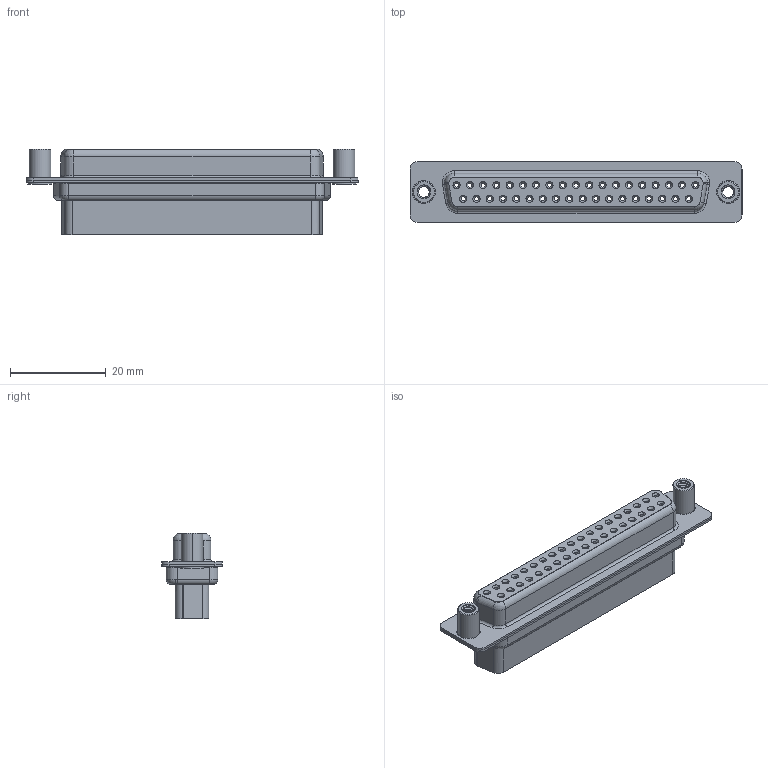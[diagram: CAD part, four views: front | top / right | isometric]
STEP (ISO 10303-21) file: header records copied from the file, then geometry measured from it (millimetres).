
FILE_DESCRIPTION (( 'STEP AP203' ), '1' );
FILE_NAME ('628-050-010-330.STEP', '2018-11-21T22:18:59', ( '' ), ( '' ), 'SwSTEP 2.0', 'SolidWorks 2016', '' );
FILE_SCHEMA (( 'CONFIG_CONTROL_DESIGN' ));
Length unit declared in the file: millimetre
Products named in the file (5): 628 Housing_37 HP; 628 Shell Front_37 Contacts; 628 Shell Rear_37 Contacts; 628 4-40 Threaded Standoff; 628-050-010-330
Assembly tree (5 placements, depth 2):
  628-050-010-330
    628 Housing_37 HP
    628 Shell Front_37 Contacts
    628 Shell Rear_37 Contacts
    628 4-40 Threaded Standoff  x2
Bounding box: 69.3 x 12.6 x 17.9 mm (x, y, z)
Volume: 6728.5 mm3; surface area: 11153.1 mm2
Topology: 5 solids, 5 shells, 794 faces, 1815 edges, 1155 vertices
Faces by surface type: cylinder 461, plane 180, cone 84, torus 63, bspline 6
Entity records: 23558 total; most frequent: CARTESIAN_POINT 5481, DIRECTION 4035, ORIENTED_EDGE 3374, AXIS2_PLACEMENT_3D 1702, EDGE_CURVE 1687, VERTEX_POINT 1072, CIRCLE 953, EDGE_LOOP 953
